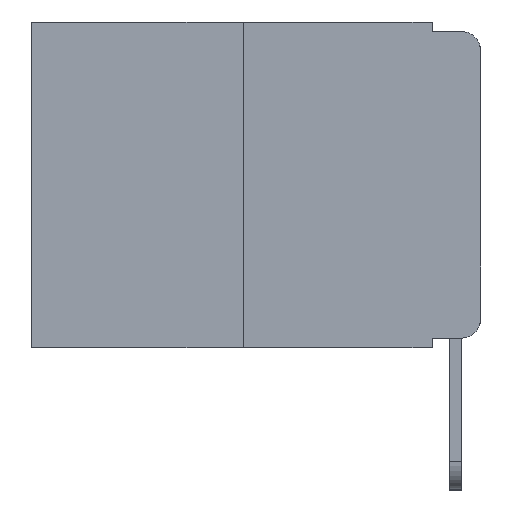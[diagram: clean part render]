
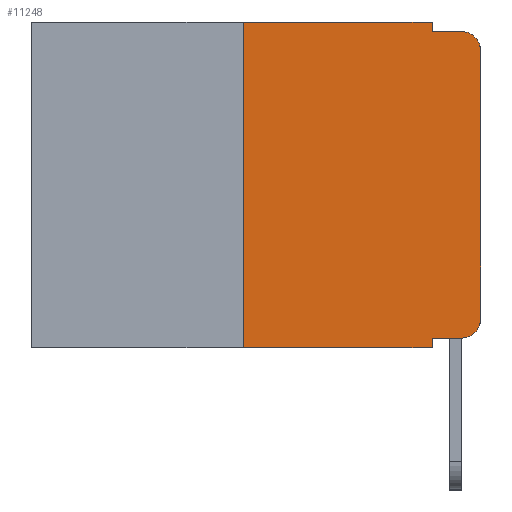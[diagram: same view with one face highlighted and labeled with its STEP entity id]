
A CAD part, left-side view. The second image highlights one B-rep face of the part: STEP entity #11248.
In plain terms, the highlighted planar face has unit normal (-1, 0, 0).
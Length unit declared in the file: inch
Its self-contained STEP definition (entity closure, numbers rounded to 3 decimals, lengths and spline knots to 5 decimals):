
#89 = LINE ( 'NONE', #11389, #1825 ) ;
#91 = ORIENTED_EDGE ( 'NONE', *, *, #488, .T. ) ;
#99 = VECTOR ( 'NONE', #9245, 39.37008 ) ;
#126 = EDGE_CURVE ( 'NONE', #11270, #12244, #14177, .T. ) ;
#373 = ORIENTED_EDGE ( 'NONE', *, *, #3920, .F. ) ;
#435 = EDGE_CURVE ( 'NONE', #13924, #7131, #17379, .T. ) ;
#488 = EDGE_CURVE ( 'NONE', #13924, #6866, #7469, .T. ) ;
#607 = AXIS2_PLACEMENT_3D ( 'NONE', #1730, #16892, #12917 ) ;
#744 = VERTEX_POINT ( 'NONE', #4656 ) ;
#929 = DIRECTION ( 'NONE',  ( 0., 0., -1. ) ) ;
#1730 = CARTESIAN_POINT ( 'NONE',  ( 0., 0.02, -0.313 ) ) ;
#1825 = VECTOR ( 'NONE', #13849, 39.37008 ) ;
#2050 = CARTESIAN_POINT ( 'NONE',  ( 0., 0.473, 0. ) ) ;
#2406 = ORIENTED_EDGE ( 'NONE', *, *, #14961, .T. ) ;
#2848 = EDGE_LOOP ( 'NONE', ( #13309, #6795, #9922, #16669, #9033, #373, #13244, #9209, #91, #2406 ) ) ;
#3727 = CARTESIAN_POINT ( 'NONE',  ( 0., 0., 0. ) ) ;
#3920 = EDGE_CURVE ( 'NONE', #744, #11270, #6907, .T. ) ;
#4435 = VECTOR ( 'NONE', #17558, 39.37008 ) ;
#4626 = VERTEX_POINT ( 'NONE', #17187 ) ;
#4656 = CARTESIAN_POINT ( 'NONE',  ( 0., 0.25, -0.343 ) ) ;
#4884 = LINE ( 'NONE', #3727, #4435 ) ;
#5032 = VERTEX_POINT ( 'NONE', #15402 ) ;
#5756 = DIRECTION ( 'NONE',  ( 0., 0., -1. ) ) ;
#6033 = CARTESIAN_POINT ( 'NONE',  ( 0., 0.051, 0. ) ) ;
#6209 = DIRECTION ( 'NONE',  ( 0., -1., 0. ) ) ;
#6387 = LINE ( 'NONE', #14180, #8166 ) ;
#6577 = CARTESIAN_POINT ( 'NONE',  ( 0., 0.473, 0. ) ) ;
#6795 = ORIENTED_EDGE ( 'NONE', *, *, #14313, .T. ) ;
#6866 = VERTEX_POINT ( 'NONE', #17666 ) ;
#6907 = LINE ( 'NONE', #13009, #8021 ) ;
#6973 = AXIS2_PLACEMENT_3D ( 'NONE', #13978, #8315, #9650 ) ;
#7131 = VERTEX_POINT ( 'NONE', #14693 ) ;
#7455 = CARTESIAN_POINT ( 'NONE',  ( 0., 0.051, -0.333 ) ) ;
#7469 = LINE ( 'NONE', #9379, #99 ) ;
#7532 = CARTESIAN_POINT ( 'NONE',  ( 0., 0.051, -0.01 ) ) ;
#7557 = EDGE_CURVE ( 'NONE', #17550, #5032, #4884, .T. ) ;
#8021 = VECTOR ( 'NONE', #14407, 39.37008 ) ;
#8042 = CIRCLE ( 'NONE', #607, 0.02 ) ;
#8166 = VECTOR ( 'NONE', #5756, 39.37008 ) ;
#8315 = DIRECTION ( 'NONE',  ( -1., 0., 0. ) ) ;
#8531 = EDGE_CURVE ( 'NONE', #744, #7131, #89, .T. ) ;
#8972 = VECTOR ( 'NONE', #10219, 39.37008 ) ;
#9027 = EDGE_CURVE ( 'NONE', #13761, #4626, #10928, .T. ) ;
#9033 = ORIENTED_EDGE ( 'NONE', *, *, #126, .F. ) ;
#9209 = ORIENTED_EDGE ( 'NONE', *, *, #435, .F. ) ;
#9245 = DIRECTION ( 'NONE',  ( 0., -1., 0. ) ) ;
#9379 = CARTESIAN_POINT ( 'NONE',  ( 0., 0.051, -0.333 ) ) ;
#9650 = DIRECTION ( 'NONE',  ( 0., 0., -1. ) ) ;
#9922 = ORIENTED_EDGE ( 'NONE', *, *, #9027, .F. ) ;
#10219 = DIRECTION ( 'NONE',  ( 0., -1., 0. ) ) ;
#10928 = LINE ( 'NONE', #7532, #8972 ) ;
#11248 = ADVANCED_FACE ( 'NONE', ( #14282 ), #17621, .F. ) ;
#11270 = VERTEX_POINT ( 'NONE', #14889 ) ;
#11389 = CARTESIAN_POINT ( 'NONE',  ( 0., 0.473, -0.343 ) ) ;
#11715 = CARTESIAN_POINT ( 'NONE',  ( 0., 0., -0.313 ) ) ;
#12012 = CARTESIAN_POINT ( 'NONE',  ( 0., 0.051, 0. ) ) ;
#12244 = VERTEX_POINT ( 'NONE', #6033 ) ;
#12585 = CIRCLE ( 'NONE', #6973, 0.02 ) ;
#12917 = DIRECTION ( 'NONE',  ( 0., 0., -1. ) ) ;
#13009 = CARTESIAN_POINT ( 'NONE',  ( 0., 0.25, 0. ) ) ;
#13244 = ORIENTED_EDGE ( 'NONE', *, *, #8531, .T. ) ;
#13309 = ORIENTED_EDGE ( 'NONE', *, *, #7557, .T. ) ;
#13761 = VERTEX_POINT ( 'NONE', #15152 ) ;
#13849 = DIRECTION ( 'NONE',  ( 0., -1., 0. ) ) ;
#13924 = VERTEX_POINT ( 'NONE', #7455 ) ;
#13965 = VECTOR ( 'NONE', #929, 39.37008 ) ;
#13978 = CARTESIAN_POINT ( 'NONE',  ( 0., 0.02, -0.03 ) ) ;
#14177 = LINE ( 'NONE', #2050, #15058 ) ;
#14180 = CARTESIAN_POINT ( 'NONE',  ( 0., 0.051, 0. ) ) ;
#14282 = FACE_OUTER_BOUND ( 'NONE', #2848, .T. ) ;
#14313 = EDGE_CURVE ( 'NONE', #5032, #4626, #12585, .T. ) ;
#14407 = DIRECTION ( 'NONE',  ( 0., 0., 1. ) ) ;
#14693 = CARTESIAN_POINT ( 'NONE',  ( 0., 0.051, -0.343 ) ) ;
#14732 = AXIS2_PLACEMENT_3D ( 'NONE', #6577, #16256, #16370 ) ;
#14889 = CARTESIAN_POINT ( 'NONE',  ( 0., 0.25, 0. ) ) ;
#14961 = EDGE_CURVE ( 'NONE', #6866, #17550, #8042, .T. ) ;
#15058 = VECTOR ( 'NONE', #6209, 39.37008 ) ;
#15152 = CARTESIAN_POINT ( 'NONE',  ( 0., 0.051, -0.01 ) ) ;
#15402 = CARTESIAN_POINT ( 'NONE',  ( 0., 0., -0.03 ) ) ;
#16256 = DIRECTION ( 'NONE',  ( 1., 0., 0. ) ) ;
#16370 = DIRECTION ( 'NONE',  ( 0., 0., -1. ) ) ;
#16669 = ORIENTED_EDGE ( 'NONE', *, *, #17397, .F. ) ;
#16892 = DIRECTION ( 'NONE',  ( -1., 0., 0. ) ) ;
#17187 = CARTESIAN_POINT ( 'NONE',  ( 0., 0.02, -0.01 ) ) ;
#17379 = LINE ( 'NONE', #12012, #13965 ) ;
#17397 = EDGE_CURVE ( 'NONE', #12244, #13761, #6387, .T. ) ;
#17550 = VERTEX_POINT ( 'NONE', #11715 ) ;
#17558 = DIRECTION ( 'NONE',  ( 0., 0., 1. ) ) ;
#17621 = PLANE ( 'NONE',  #14732 ) ;
#17666 = CARTESIAN_POINT ( 'NONE',  ( 0., 0.02, -0.333 ) ) ;
